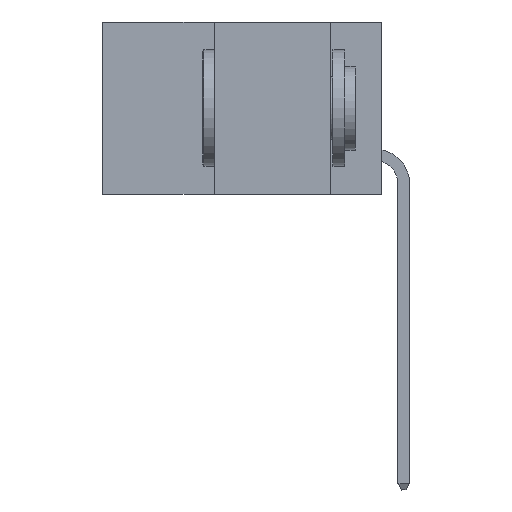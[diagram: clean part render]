
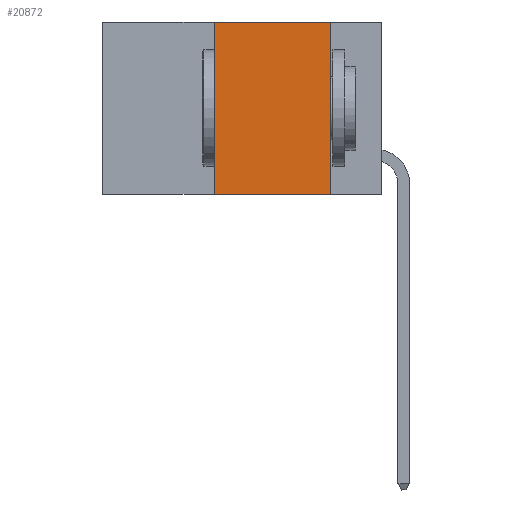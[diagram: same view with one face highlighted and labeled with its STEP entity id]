
A CAD part, left-side view. The second image highlights one B-rep face of the part: STEP entity #20872.
In plain terms, the highlighted planar face has unit normal (-1, 0, 0).
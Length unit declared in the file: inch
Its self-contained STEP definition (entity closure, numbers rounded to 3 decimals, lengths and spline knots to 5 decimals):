
#1623 = CARTESIAN_POINT ( 'NONE',  ( 0., 0.36, 0. ) ) ;
#1989 = EDGE_CURVE ( 'NONE', #10099, #6304, #3664, .T. ) ;
#2178 = CARTESIAN_POINT ( 'NONE',  ( 0., 0.6, 0. ) ) ;
#2682 = VECTOR ( 'NONE', #22045, 39.37008 ) ;
#2892 = CARTESIAN_POINT ( 'NONE',  ( 0., 0.11, 0. ) ) ;
#3664 = LINE ( 'NONE', #2892, #2682 ) ;
#5436 = LINE ( 'NONE', #22190, #10406 ) ;
#6304 = VERTEX_POINT ( 'NONE', #22138 ) ;
#6631 = EDGE_LOOP ( 'NONE', ( #8193, #23981, #24514, #7281 ) ) ;
#7281 = ORIENTED_EDGE ( 'NONE', *, *, #20366, .T. ) ;
#7778 = EDGE_CURVE ( 'NONE', #9912, #15285, #21525, .T. ) ;
#8193 = ORIENTED_EDGE ( 'NONE', *, *, #1989, .F. ) ;
#8524 = CARTESIAN_POINT ( 'NONE',  ( 0., 0.36, -0.37 ) ) ;
#9912 = VERTEX_POINT ( 'NONE', #8524 ) ;
#10099 = VERTEX_POINT ( 'NONE', #22124 ) ;
#10406 = VECTOR ( 'NONE', #26474, 39.37008 ) ;
#11611 = PLANE ( 'NONE',  #19380 ) ;
#12183 = CARTESIAN_POINT ( 'NONE',  ( 0., 0.36, 0. ) ) ;
#12580 = DIRECTION ( 'NONE',  ( 0., -1., 0. ) ) ;
#15285 = VERTEX_POINT ( 'NONE', #1623 ) ;
#18093 = DIRECTION ( 'NONE',  ( 1., 0., 0. ) ) ;
#19380 = AXIS2_PLACEMENT_3D ( 'NONE', #26250, #18093, #24566 ) ;
#20037 = FACE_OUTER_BOUND ( 'NONE', #6631, .T. ) ;
#20366 = EDGE_CURVE ( 'NONE', #9912, #6304, #5436, .T. ) ;
#20872 = ADVANCED_FACE ( 'NONE', ( #20037 ), #11611, .F. ) ;
#21525 = LINE ( 'NONE', #12183, #24519 ) ;
#21616 = LINE ( 'NONE', #2178, #22333 ) ;
#21816 = EDGE_CURVE ( 'NONE', #15285, #10099, #21616, .T. ) ;
#22045 = DIRECTION ( 'NONE',  ( 0., 0., -1. ) ) ;
#22124 = CARTESIAN_POINT ( 'NONE',  ( 0., 0.11, 0. ) ) ;
#22138 = CARTESIAN_POINT ( 'NONE',  ( 0., 0.11, -0.37 ) ) ;
#22190 = CARTESIAN_POINT ( 'NONE',  ( 0., 0.6, -0.37 ) ) ;
#22333 = VECTOR ( 'NONE', #12580, 39.37008 ) ;
#22821 = DIRECTION ( 'NONE',  ( 0., 0., 1. ) ) ;
#23981 = ORIENTED_EDGE ( 'NONE', *, *, #21816, .F. ) ;
#24514 = ORIENTED_EDGE ( 'NONE', *, *, #7778, .F. ) ;
#24519 = VECTOR ( 'NONE', #22821, 39.37008 ) ;
#24566 = DIRECTION ( 'NONE',  ( 0., 0., -1. ) ) ;
#26250 = CARTESIAN_POINT ( 'NONE',  ( 0., 0.6, 0. ) ) ;
#26474 = DIRECTION ( 'NONE',  ( 0., -1., 0. ) ) ;
